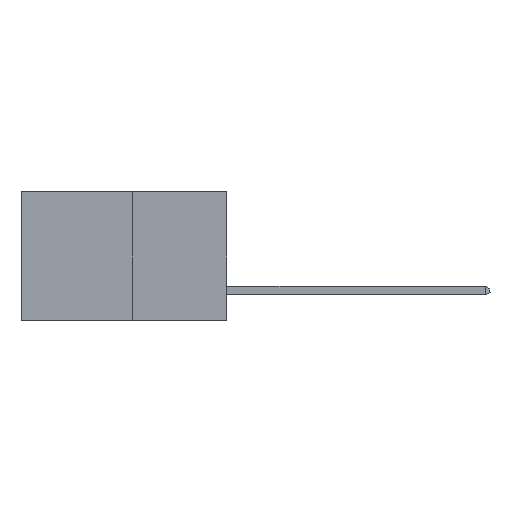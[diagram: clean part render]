
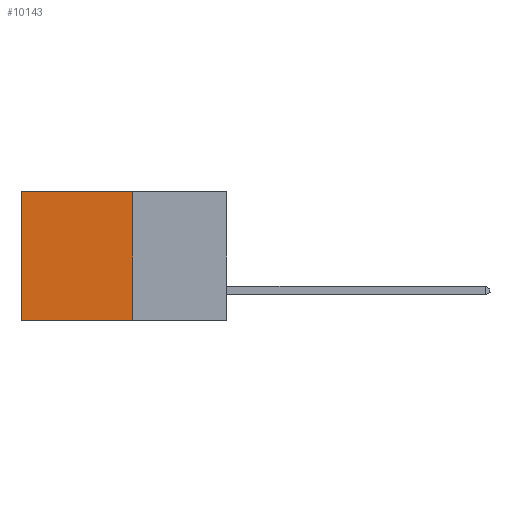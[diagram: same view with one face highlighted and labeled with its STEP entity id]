
A CAD part, left-side view. The second image highlights one B-rep face of the part: STEP entity #10143.
In plain terms, the highlighted planar face has unit normal (-1, 0, 0).
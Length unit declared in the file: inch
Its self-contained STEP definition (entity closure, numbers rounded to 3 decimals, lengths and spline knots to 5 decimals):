
#798 = EDGE_CURVE ( 'NONE', #3589, #15605, #9150, .T. ) ;
#844 = FACE_OUTER_BOUND ( 'NONE', #1625, .T. ) ;
#852 = CARTESIAN_POINT ( 'NONE',  ( 0.277, 0.27, -0.37 ) ) ;
#911 = LINE ( 'NONE', #1286, #6694 ) ;
#1286 = CARTESIAN_POINT ( 'NONE',  ( 0.277, 0.59, -0.37 ) ) ;
#1366 = ORIENTED_EDGE ( 'NONE', *, *, #5749, .T. ) ;
#1625 = EDGE_LOOP ( 'NONE', ( #1366, #8266, #11933, #15109 ) ) ;
#1631 = CARTESIAN_POINT ( 'NONE',  ( 0.277, 0.59, -0.37 ) ) ;
#2713 = VERTEX_POINT ( 'NONE', #1631 ) ;
#3182 = DIRECTION ( 'NONE',  ( 0., 1., 0. ) ) ;
#3589 = VERTEX_POINT ( 'NONE', #15506 ) ;
#4108 = AXIS2_PLACEMENT_3D ( 'NONE', #6018, #14499, #7220 ) ;
#5014 = VECTOR ( 'NONE', #3182, 39.37008 ) ;
#5749 = EDGE_CURVE ( 'NONE', #14758, #2713, #911, .T. ) ;
#6018 = CARTESIAN_POINT ( 'NONE',  ( 0.277, 0.27, -0.37 ) ) ;
#6694 = VECTOR ( 'NONE', #12862, 39.37008 ) ;
#6852 = DIRECTION ( 'NONE',  ( 0., 0., -1. ) ) ;
#7220 = DIRECTION ( 'NONE',  ( 0., 0., -1. ) ) ;
#7431 = CARTESIAN_POINT ( 'NONE',  ( 0.277, 0.59, 0. ) ) ;
#7575 = EDGE_CURVE ( 'NONE', #3589, #14758, #11240, .T. ) ;
#8193 = CARTESIAN_POINT ( 'NONE',  ( 0.277, 0.27, 0. ) ) ;
#8266 = ORIENTED_EDGE ( 'NONE', *, *, #13301, .F. ) ;
#9150 = LINE ( 'NONE', #852, #15234 ) ;
#9395 = DIRECTION ( 'NONE',  ( 0., 1., 0. ) ) ;
#10143 = ADVANCED_FACE ( 'NONE', ( #844 ), #13330, .F. ) ;
#11240 = LINE ( 'NONE', #8193, #14806 ) ;
#11504 = LINE ( 'NONE', #14124, #5014 ) ;
#11531 = CARTESIAN_POINT ( 'NONE',  ( 0.277, 0.27, -0.37 ) ) ;
#11933 = ORIENTED_EDGE ( 'NONE', *, *, #798, .F. ) ;
#12862 = DIRECTION ( 'NONE',  ( 0., 0., -1. ) ) ;
#13301 = EDGE_CURVE ( 'NONE', #15605, #2713, #11504, .T. ) ;
#13330 = PLANE ( 'NONE',  #4108 ) ;
#14124 = CARTESIAN_POINT ( 'NONE',  ( 0.277, 0.27, -0.37 ) ) ;
#14499 = DIRECTION ( 'NONE',  ( 1., 0., 0. ) ) ;
#14758 = VERTEX_POINT ( 'NONE', #7431 ) ;
#14806 = VECTOR ( 'NONE', #9395, 39.37008 ) ;
#15109 = ORIENTED_EDGE ( 'NONE', *, *, #7575, .T. ) ;
#15234 = VECTOR ( 'NONE', #6852, 39.37008 ) ;
#15506 = CARTESIAN_POINT ( 'NONE',  ( 0.277, 0.27, 0. ) ) ;
#15605 = VERTEX_POINT ( 'NONE', #11531 ) ;
